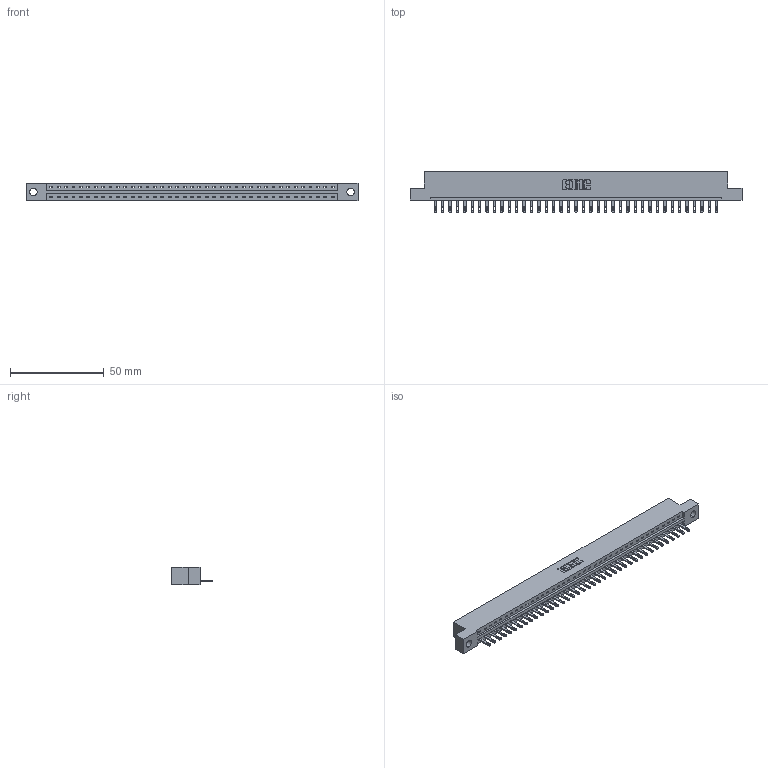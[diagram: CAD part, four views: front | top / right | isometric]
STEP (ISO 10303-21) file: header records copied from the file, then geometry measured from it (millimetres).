
FILE_DESCRIPTION (( 'STEP AP203' ), '1' );
FILE_NAME ('337-039-500-104.STEP', '2019-10-01T17:54:55', ( '' ), ( '' ), 'SwSTEP 2.0', 'SolidWorks 2016', '' );
FILE_SCHEMA (( 'CONFIG_CONTROL_DESIGN' ));
Length unit declared in the file: inch
Products named in the file (3): 345-292-001_345-293-100; 337-039-500-104; 337 Part_Flush Mounting Lugs - 0.156 Dia-TH
Assembly tree (40 placements, depth 2):
  337-039-500-104
    337 Part_Flush Mounting Lugs - 0.156 Dia-TH
    345-292-001_345-293-100  x39
Bounding box: 177.55 x 21.85 x 9.4 mm (x, y, z)
Volume: 18351.7 mm3; surface area: 18833.4 mm2
Topology: 40 solids, 40 shells, 2376 faces, 7331 edges, 4886 vertices
Faces by surface type: plane 1630, cylinder 746
Entity records: 29311 total; most frequent: CARTESIAN_POINT 5111, ORIENTED_EDGE 5086, DIRECTION 4309, EDGE_CURVE 2543, VECTOR 2411, LINE 2411, VERTEX_POINT 1694, AXIS2_PLACEMENT_3D 949
